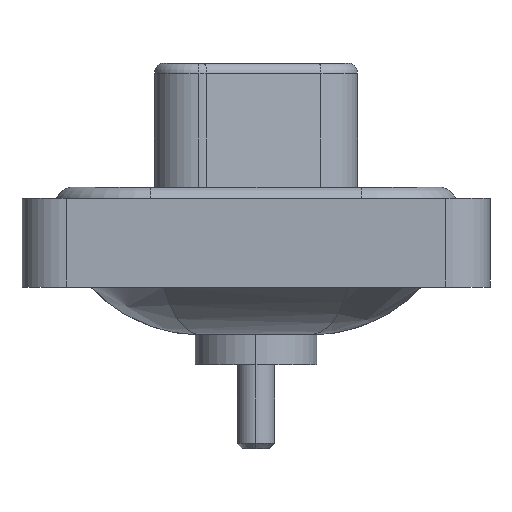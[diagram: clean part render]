
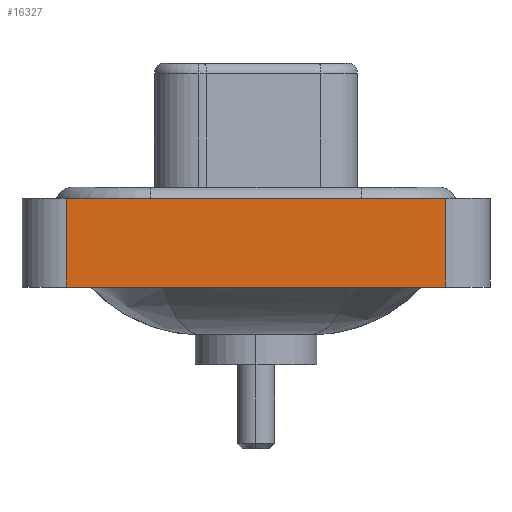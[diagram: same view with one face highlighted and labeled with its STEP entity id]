
A CAD part, left-side view. The second image highlights one B-rep face of the part: STEP entity #16327.
In plain terms, the highlighted planar face has unit normal (-1, 0, 0).
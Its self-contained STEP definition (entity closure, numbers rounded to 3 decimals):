
#2 = DIRECTION ( 'NONE',  ( 0., 0., 1. ) ) ;
#1098 = VECTOR ( 'NONE', #2, 1000. ) ;
#1930 = ORIENTED_EDGE ( 'NONE', *, *, #9865, .F. ) ;
#2192 = DIRECTION ( 'NONE',  ( 0., 0., 1. ) ) ;
#2579 = EDGE_CURVE ( 'NONE', #6902, #2658, #12785, .T. ) ;
#2658 = VERTEX_POINT ( 'NONE', #15254 ) ;
#3540 = EDGE_CURVE ( 'NONE', #2658, #9377, #11745, .T. ) ;
#3766 = CARTESIAN_POINT ( 'NONE',  ( -7.3, 8.55, -3.6 ) ) ;
#4219 = VECTOR ( 'NONE', #6644, 1000. ) ;
#5319 = DIRECTION ( 'NONE',  ( -1., 0., 0. ) ) ;
#5822 = LINE ( 'NONE', #12052, #13571 ) ;
#6303 = VECTOR ( 'NONE', #2192, 1000. ) ;
#6644 = DIRECTION ( 'NONE',  ( 0., -1., 0. ) ) ;
#6760 = CARTESIAN_POINT ( 'NONE',  ( -7.3, 8.55, -3.6 ) ) ;
#6902 = VERTEX_POINT ( 'NONE', #6760 ) ;
#7714 = ORIENTED_EDGE ( 'NONE', *, *, #3540, .T. ) ;
#7946 = CARTESIAN_POINT ( 'NONE',  ( -7.3, 8.55, 0.4 ) ) ;
#8473 = CARTESIAN_POINT ( 'NONE',  ( -7.3, -8.55, 0.4 ) ) ;
#9377 = VERTEX_POINT ( 'NONE', #8473 ) ;
#9865 = EDGE_CURVE ( 'NONE', #15089, #9377, #5822, .T. ) ;
#10274 = CARTESIAN_POINT ( 'NONE',  ( -7.3, -8.55, -3.6 ) ) ;
#10892 = LINE ( 'NONE', #3766, #6303 ) ;
#11260 = DIRECTION ( 'NONE',  ( 0., 0., 1. ) ) ;
#11449 = PLANE ( 'NONE',  #14628 ) ;
#11745 = LINE ( 'NONE', #10274, #1098 ) ;
#12052 = CARTESIAN_POINT ( 'NONE',  ( -7.3, -8.55, 0.4 ) ) ;
#12785 = LINE ( 'NONE', #15544, #4219 ) ;
#13571 = VECTOR ( 'NONE', #19332, 1000. ) ;
#14628 = AXIS2_PLACEMENT_3D ( 'NONE', #17431, #5319, #11260 ) ;
#14695 = EDGE_CURVE ( 'NONE', #6902, #15089, #10892, .T. ) ;
#15089 = VERTEX_POINT ( 'NONE', #7946 ) ;
#15239 = EDGE_LOOP ( 'NONE', ( #7714, #1930, #16506, #15841 ) ) ;
#15254 = CARTESIAN_POINT ( 'NONE',  ( -7.3, -8.55, -3.6 ) ) ;
#15544 = CARTESIAN_POINT ( 'NONE',  ( -7.3, -8.55, -3.6 ) ) ;
#15841 = ORIENTED_EDGE ( 'NONE', *, *, #2579, .T. ) ;
#16327 = ADVANCED_FACE ( 'NONE', ( #18822 ), #11449, .T. ) ;
#16506 = ORIENTED_EDGE ( 'NONE', *, *, #14695, .F. ) ;
#17431 = CARTESIAN_POINT ( 'NONE',  ( -7.3, -8.55, -3.6 ) ) ;
#18822 = FACE_OUTER_BOUND ( 'NONE', #15239, .T. ) ;
#19332 = DIRECTION ( 'NONE',  ( 0., -1., 0. ) ) ;
